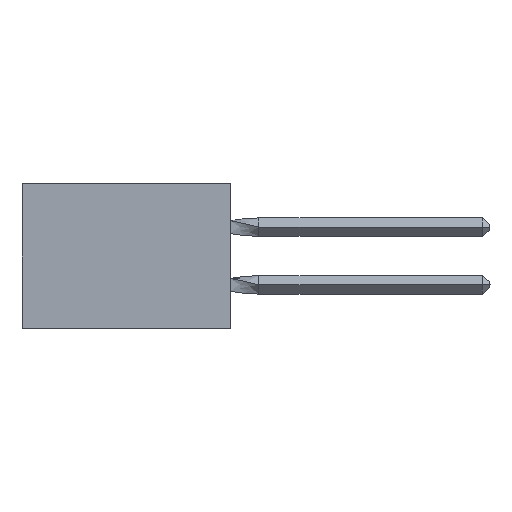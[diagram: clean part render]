
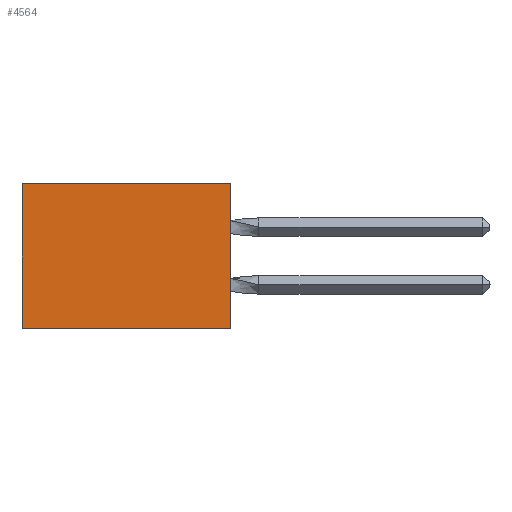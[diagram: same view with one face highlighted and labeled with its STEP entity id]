
A CAD part, left-side view. The second image highlights one B-rep face of the part: STEP entity #4564.
In plain terms, the highlighted planar face has unit normal (-1, 0, 0).
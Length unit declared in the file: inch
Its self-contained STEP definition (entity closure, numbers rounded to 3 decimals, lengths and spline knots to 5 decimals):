
#579 = EDGE_CURVE ( 'NONE', #12720, #3916, #12776, .T. ) ;
#594 = LINE ( 'NONE', #11734, #14241 ) ;
#1702 = CARTESIAN_POINT ( 'NONE',  ( 0.305, 0., 0. ) ) ;
#1717 = VERTEX_POINT ( 'NONE', #8297 ) ;
#2462 = EDGE_CURVE ( 'NONE', #3807, #1717, #594, .T. ) ;
#2728 = ORIENTED_EDGE ( 'NONE', *, *, #2462, .F. ) ;
#2968 = CARTESIAN_POINT ( 'NONE',  ( 0.305, 0., -0.5 ) ) ;
#3206 = CARTESIAN_POINT ( 'NONE',  ( 0.305, 0.72, 0. ) ) ;
#3807 = VERTEX_POINT ( 'NONE', #15906 ) ;
#3916 = VERTEX_POINT ( 'NONE', #12458 ) ;
#4564 = ADVANCED_FACE ( 'NONE', ( #10364 ), #12683, .F. ) ;
#4786 = DIRECTION ( 'NONE',  ( 0., 1., 0. ) ) ;
#5453 = DIRECTION ( 'NONE',  ( 0., 0., -1. ) ) ;
#6618 = CARTESIAN_POINT ( 'NONE',  ( 0.305, 0.72, -0.5 ) ) ;
#6702 = DIRECTION ( 'NONE',  ( 1., 0., 0. ) ) ;
#7493 = VECTOR ( 'NONE', #13979, 39.37008 ) ;
#7880 = DIRECTION ( 'NONE',  ( 0., 0., -1. ) ) ;
#8297 = CARTESIAN_POINT ( 'NONE',  ( 0.305, 0., -0.5 ) ) ;
#8375 = CARTESIAN_POINT ( 'NONE',  ( 0.305, 0., -0.5 ) ) ;
#8841 = LINE ( 'NONE', #8375, #15733 ) ;
#9216 = EDGE_CURVE ( 'NONE', #1717, #3916, #8841, .T. ) ;
#9571 = ORIENTED_EDGE ( 'NONE', *, *, #15897, .T. ) ;
#10011 = ORIENTED_EDGE ( 'NONE', *, *, #579, .T. ) ;
#10190 = ORIENTED_EDGE ( 'NONE', *, *, #9216, .F. ) ;
#10364 = FACE_OUTER_BOUND ( 'NONE', #15486, .T. ) ;
#11734 = CARTESIAN_POINT ( 'NONE',  ( 0.305, 0., -0.5 ) ) ;
#12458 = CARTESIAN_POINT ( 'NONE',  ( 0.305, 0.72, -0.5 ) ) ;
#12496 = LINE ( 'NONE', #1702, #7493 ) ;
#12683 = PLANE ( 'NONE',  #15451 ) ;
#12720 = VERTEX_POINT ( 'NONE', #3206 ) ;
#12776 = LINE ( 'NONE', #6618, #15821 ) ;
#13979 = DIRECTION ( 'NONE',  ( 0., 1., 0. ) ) ;
#14241 = VECTOR ( 'NONE', #15376, 39.37008 ) ;
#15376 = DIRECTION ( 'NONE',  ( 0., 0., -1. ) ) ;
#15451 = AXIS2_PLACEMENT_3D ( 'NONE', #2968, #6702, #5453 ) ;
#15486 = EDGE_LOOP ( 'NONE', ( #10011, #10190, #2728, #9571 ) ) ;
#15733 = VECTOR ( 'NONE', #4786, 39.37008 ) ;
#15821 = VECTOR ( 'NONE', #7880, 39.37008 ) ;
#15897 = EDGE_CURVE ( 'NONE', #3807, #12720, #12496, .T. ) ;
#15906 = CARTESIAN_POINT ( 'NONE',  ( 0.305, 0., 0. ) ) ;
